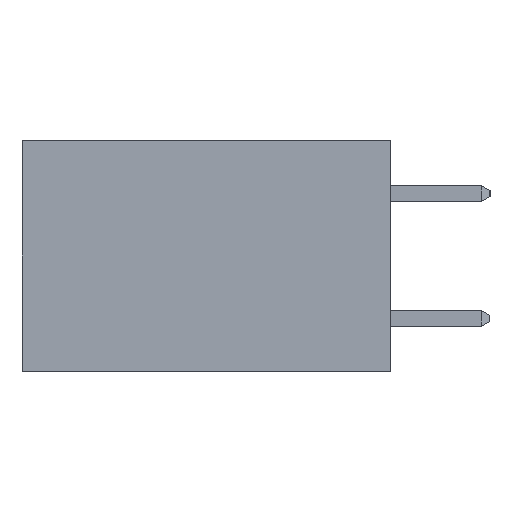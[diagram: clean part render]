
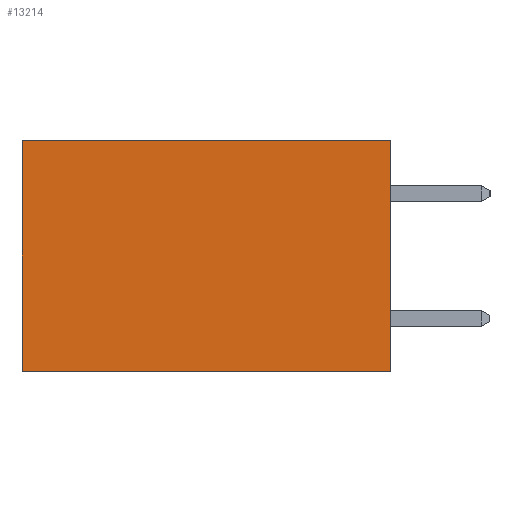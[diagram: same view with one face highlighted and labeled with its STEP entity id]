
A CAD part, left-side view. The second image highlights one B-rep face of the part: STEP entity #13214.
In plain terms, the highlighted planar face has unit normal (-1, 0, 0).
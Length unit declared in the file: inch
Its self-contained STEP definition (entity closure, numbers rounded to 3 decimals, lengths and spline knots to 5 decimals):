
#1052 = VERTEX_POINT ( 'NONE', #3975 ) ;
#1345 = EDGE_CURVE ( 'NONE', #1052, #3345, #8302, .T. ) ;
#2523 = DIRECTION ( 'NONE',  ( 0., 0., -1. ) ) ;
#3171 = ORIENTED_EDGE ( 'NONE', *, *, #1345, .F. ) ;
#3220 = CARTESIAN_POINT ( 'NONE',  ( 0.277, 0., -0.37 ) ) ;
#3303 = CARTESIAN_POINT ( 'NONE',  ( 0.277, 0., -0.37 ) ) ;
#3320 = DIRECTION ( 'NONE',  ( 0., 1., 0. ) ) ;
#3345 = VERTEX_POINT ( 'NONE', #3303 ) ;
#3509 = FACE_OUTER_BOUND ( 'NONE', #11707, .T. ) ;
#3639 = AXIS2_PLACEMENT_3D ( 'NONE', #4762, #14406, #6227 ) ;
#3975 = CARTESIAN_POINT ( 'NONE',  ( 0.277, 0., 0. ) ) ;
#4241 = LINE ( 'NONE', #7181, #14854 ) ;
#4762 = CARTESIAN_POINT ( 'NONE',  ( 0.277, 0., -0.37 ) ) ;
#4931 = VECTOR ( 'NONE', #2523, 39.37008 ) ;
#5128 = EDGE_CURVE ( 'NONE', #3345, #6115, #8877, .T. ) ;
#5358 = VERTEX_POINT ( 'NONE', #16578 ) ;
#5580 = CARTESIAN_POINT ( 'NONE',  ( 0.277, 0.59, -0.37 ) ) ;
#6115 = VERTEX_POINT ( 'NONE', #8089 ) ;
#6227 = DIRECTION ( 'NONE',  ( 0., 0., -1. ) ) ;
#7012 = DIRECTION ( 'NONE',  ( 0., 0., -1. ) ) ;
#7181 = CARTESIAN_POINT ( 'NONE',  ( 0.277, 0., 0. ) ) ;
#7458 = LINE ( 'NONE', #5580, #14236 ) ;
#8089 = CARTESIAN_POINT ( 'NONE',  ( 0.277, 0.59, -0.37 ) ) ;
#8302 = LINE ( 'NONE', #3220, #4931 ) ;
#8877 = LINE ( 'NONE', #15129, #12009 ) ;
#10302 = ORIENTED_EDGE ( 'NONE', *, *, #11951, .T. ) ;
#10719 = ORIENTED_EDGE ( 'NONE', *, *, #12974, .T. ) ;
#11707 = EDGE_LOOP ( 'NONE', ( #10302, #17669, #3171, #10719 ) ) ;
#11951 = EDGE_CURVE ( 'NONE', #5358, #6115, #7458, .T. ) ;
#12009 = VECTOR ( 'NONE', #3320, 39.37008 ) ;
#12578 = DIRECTION ( 'NONE',  ( 0., 1., 0. ) ) ;
#12974 = EDGE_CURVE ( 'NONE', #1052, #5358, #4241, .T. ) ;
#13023 = PLANE ( 'NONE',  #3639 ) ;
#13214 = ADVANCED_FACE ( 'NONE', ( #3509 ), #13023, .F. ) ;
#14236 = VECTOR ( 'NONE', #7012, 39.37008 ) ;
#14406 = DIRECTION ( 'NONE',  ( 1., 0., 0. ) ) ;
#14854 = VECTOR ( 'NONE', #12578, 39.37008 ) ;
#15129 = CARTESIAN_POINT ( 'NONE',  ( 0.277, 0., -0.37 ) ) ;
#16578 = CARTESIAN_POINT ( 'NONE',  ( 0.277, 0.59, 0. ) ) ;
#17669 = ORIENTED_EDGE ( 'NONE', *, *, #5128, .F. ) ;
